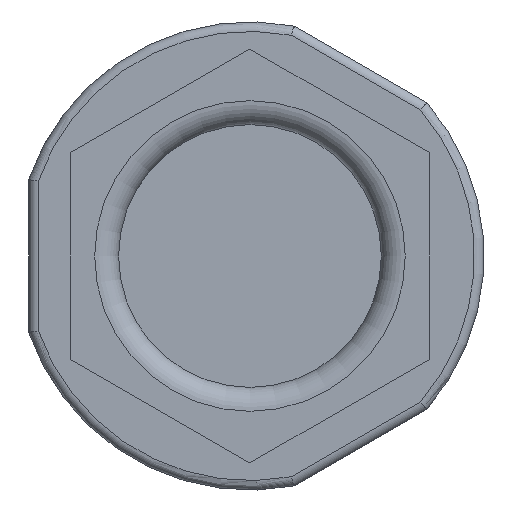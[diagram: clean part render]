
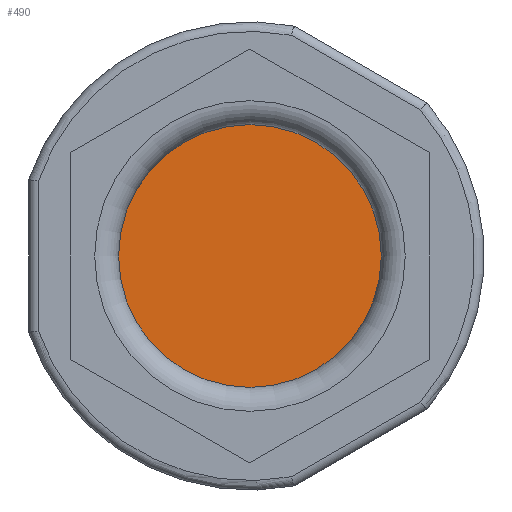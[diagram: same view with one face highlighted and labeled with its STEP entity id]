
A CAD part, front view. The second image highlights one B-rep face of the part: STEP entity #490.
In plain terms, the highlighted planar face has unit normal (0, -1, 0).
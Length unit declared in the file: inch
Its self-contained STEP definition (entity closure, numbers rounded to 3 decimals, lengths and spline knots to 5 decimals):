
#125=FACE_OUTER_BOUND('',#158,.T.);
#158=EDGE_LOOP('',(#332));
#194=CIRCLE('',#538,0.275);
#216=VERTEX_POINT('',#741);
#260=EDGE_CURVE('',#216,#216,#194,.T.);
#332=ORIENTED_EDGE('',*,*,#260,.F.);
#476=PLANE('',#537);
#490=ADVANCED_FACE('',(#125),#476,.T.);
#537=AXIS2_PLACEMENT_3D('',#740,#593,#594);
#538=AXIS2_PLACEMENT_3D('',#742,#595,#596);
#593=DIRECTION('center_axis',(0.,-1.,0.));
#594=DIRECTION('ref_axis',(1.,0.,0.));
#595=DIRECTION('center_axis',(0.,1.,0.));
#596=DIRECTION('ref_axis',(1.,0.,0.));
#740=CARTESIAN_POINT('Origin',(0.,2.94425,0.));
#741=CARTESIAN_POINT('',(-0.275,2.94425,0.));
#742=CARTESIAN_POINT('Origin',(0.,2.94425,0.));
